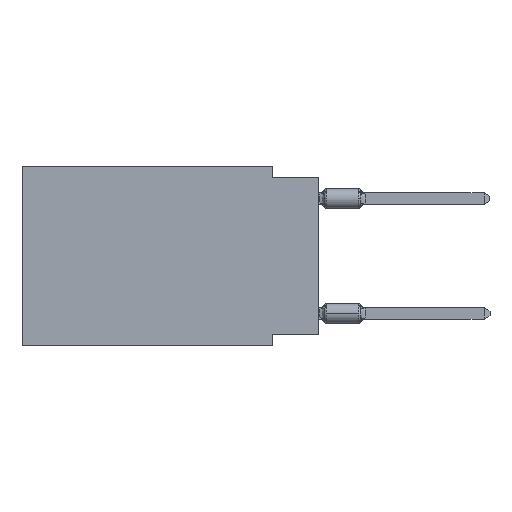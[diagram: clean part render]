
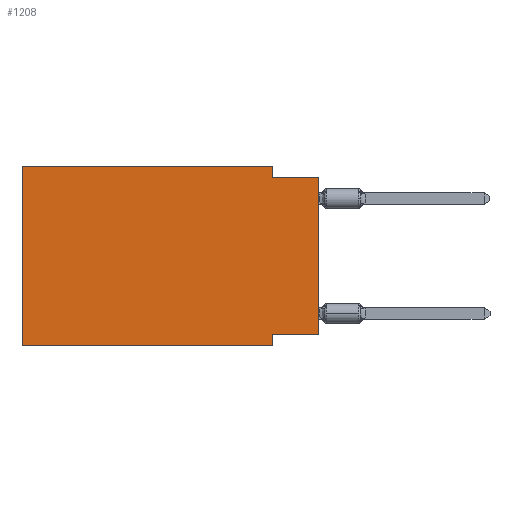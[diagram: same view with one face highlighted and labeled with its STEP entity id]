
A CAD part, left-side view. The second image highlights one B-rep face of the part: STEP entity #1208.
In plain terms, the highlighted planar face has unit normal (-1, 0, 0).
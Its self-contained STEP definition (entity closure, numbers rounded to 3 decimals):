
#7 = PLANE ( 'NONE',  #43 ) ;
#43 = AXIS2_PLACEMENT_3D ( 'NONE', #9394, #18500, #16987 ) ;
#185 = VERTEX_POINT ( 'NONE', #18990 ) ;
#499 = LINE ( 'NONE', #2308, #14584 ) ;
#718 = EDGE_CURVE ( 'NONE', #5437, #13035, #7610, .T. ) ;
#805 = DIRECTION ( 'NONE',  ( 0., 1., 0. ) ) ;
#1208 = ADVANCED_FACE ( 'NONE', ( #13847 ), #7, .F. ) ;
#1634 = EDGE_CURVE ( 'NONE', #10413, #5437, #499, .T. ) ;
#2123 = CARTESIAN_POINT ( 'NONE',  ( 0., 16.383, 0. ) ) ;
#2308 = CARTESIAN_POINT ( 'NONE',  ( 0., 0., -9.271 ) ) ;
#2372 = EDGE_LOOP ( 'NONE', ( #9032, #5374, #12739, #14427, #4566, #19195, #12117, #3704 ) ) ;
#2853 = LINE ( 'NONE', #18017, #14326 ) ;
#3285 = VECTOR ( 'NONE', #12069, 1000. ) ;
#3335 = CARTESIAN_POINT ( 'NONE',  ( 0., 16.383, -9.906 ) ) ;
#3357 = EDGE_CURVE ( 'NONE', #10536, #5734, #14628, .T. ) ;
#3704 = ORIENTED_EDGE ( 'NONE', *, *, #1634, .F. ) ;
#3759 = VECTOR ( 'NONE', #8483, 1000. ) ;
#4421 = LINE ( 'NONE', #10787, #19508 ) ;
#4566 = ORIENTED_EDGE ( 'NONE', *, *, #3357, .F. ) ;
#4572 = CARTESIAN_POINT ( 'NONE',  ( 0., 0., 0. ) ) ;
#4836 = EDGE_CURVE ( 'NONE', #5734, #7949, #13042, .T. ) ;
#4842 = VECTOR ( 'NONE', #15393, 1000. ) ;
#5374 = ORIENTED_EDGE ( 'NONE', *, *, #9065, .F. ) ;
#5437 = VERTEX_POINT ( 'NONE', #19651 ) ;
#5734 = VERTEX_POINT ( 'NONE', #11843 ) ;
#5861 = VECTOR ( 'NONE', #19592, 1000. ) ;
#6938 = CARTESIAN_POINT ( 'NONE',  ( 0., 16.383, 0. ) ) ;
#7404 = LINE ( 'NONE', #4572, #4842 ) ;
#7610 = LINE ( 'NONE', #13776, #3285 ) ;
#7949 = VERTEX_POINT ( 'NONE', #14334 ) ;
#8483 = DIRECTION ( 'NONE',  ( 0., -1., 0. ) ) ;
#9004 = DIRECTION ( 'NONE',  ( 0., -1., 0. ) ) ;
#9032 = ORIENTED_EDGE ( 'NONE', *, *, #11836, .T. ) ;
#9065 = EDGE_CURVE ( 'NONE', #18020, #185, #2853, .T. ) ;
#9394 = CARTESIAN_POINT ( 'NONE',  ( 0., 16.383, 0. ) ) ;
#9778 = EDGE_CURVE ( 'NONE', #10536, #13035, #4421, .T. ) ;
#10413 = VERTEX_POINT ( 'NONE', #11564 ) ;
#10536 = VERTEX_POINT ( 'NONE', #3335 ) ;
#10719 = EDGE_CURVE ( 'NONE', #7949, #18020, #13146, .T. ) ;
#10787 = CARTESIAN_POINT ( 'NONE',  ( 0., 16.383, -9.906 ) ) ;
#11564 = CARTESIAN_POINT ( 'NONE',  ( 0., 0., -9.271 ) ) ;
#11836 = EDGE_CURVE ( 'NONE', #10413, #185, #7404, .T. ) ;
#11843 = CARTESIAN_POINT ( 'NONE',  ( 0., 16.383, 0. ) ) ;
#12069 = DIRECTION ( 'NONE',  ( 0., 0., -1. ) ) ;
#12117 = ORIENTED_EDGE ( 'NONE', *, *, #718, .F. ) ;
#12739 = ORIENTED_EDGE ( 'NONE', *, *, #10719, .F. ) ;
#13035 = VERTEX_POINT ( 'NONE', #16808 ) ;
#13042 = LINE ( 'NONE', #2123, #3759 ) ;
#13146 = LINE ( 'NONE', #16283, #5861 ) ;
#13776 = CARTESIAN_POINT ( 'NONE',  ( 0., 2.54, -9.906 ) ) ;
#13847 = FACE_OUTER_BOUND ( 'NONE', #2372, .T. ) ;
#14326 = VECTOR ( 'NONE', #9004, 1000. ) ;
#14334 = CARTESIAN_POINT ( 'NONE',  ( 0., 2.54, 0. ) ) ;
#14427 = ORIENTED_EDGE ( 'NONE', *, *, #4836, .F. ) ;
#14584 = VECTOR ( 'NONE', #805, 1000. ) ;
#14628 = LINE ( 'NONE', #6938, #17040 ) ;
#15393 = DIRECTION ( 'NONE',  ( 0., 0., 1. ) ) ;
#15398 = CARTESIAN_POINT ( 'NONE',  ( 0., 2.54, -0.635 ) ) ;
#15442 = DIRECTION ( 'NONE',  ( 0., -1., 0. ) ) ;
#16283 = CARTESIAN_POINT ( 'NONE',  ( 0., 2.54, 0. ) ) ;
#16808 = CARTESIAN_POINT ( 'NONE',  ( 0., 2.54, -9.906 ) ) ;
#16987 = DIRECTION ( 'NONE',  ( 0., 0., -1. ) ) ;
#17040 = VECTOR ( 'NONE', #17349, 1000. ) ;
#17349 = DIRECTION ( 'NONE',  ( 0., 0., 1. ) ) ;
#18017 = CARTESIAN_POINT ( 'NONE',  ( 0., 0., -0.635 ) ) ;
#18020 = VERTEX_POINT ( 'NONE', #15398 ) ;
#18500 = DIRECTION ( 'NONE',  ( 1., 0., 0. ) ) ;
#18990 = CARTESIAN_POINT ( 'NONE',  ( 0., 0., -0.635 ) ) ;
#19195 = ORIENTED_EDGE ( 'NONE', *, *, #9778, .T. ) ;
#19508 = VECTOR ( 'NONE', #15442, 1000. ) ;
#19592 = DIRECTION ( 'NONE',  ( 0., 0., -1. ) ) ;
#19651 = CARTESIAN_POINT ( 'NONE',  ( 0., 2.54, -9.271 ) ) ;
